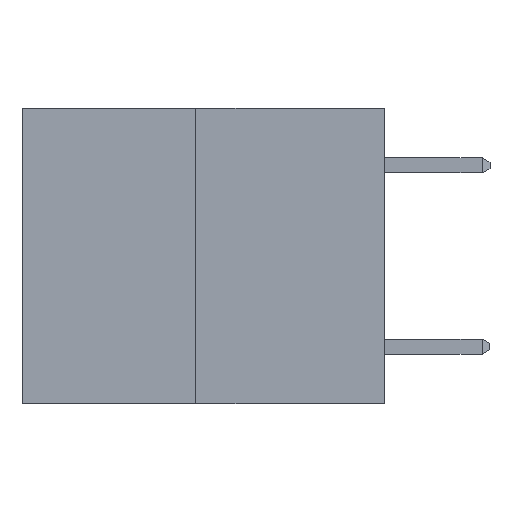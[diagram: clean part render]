
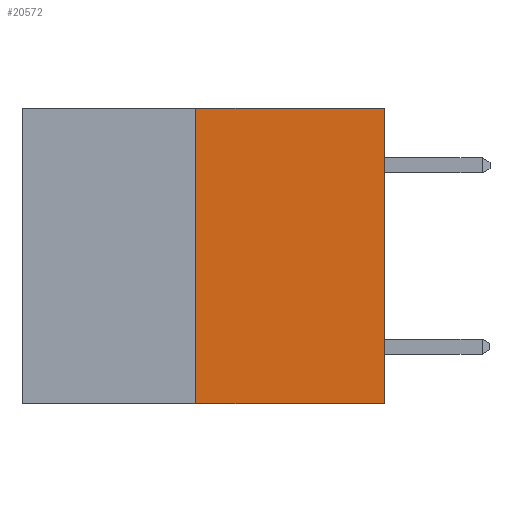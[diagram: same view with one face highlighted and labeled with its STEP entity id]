
A CAD part, left-side view. The second image highlights one B-rep face of the part: STEP entity #20572.
In plain terms, the highlighted planar face has unit normal (-1, 0, 0).
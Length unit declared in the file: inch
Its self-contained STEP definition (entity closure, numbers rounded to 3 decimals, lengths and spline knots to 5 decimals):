
#237 = EDGE_CURVE ( 'NONE', #17981, #3026, #12383, .T. ) ;
#826 = CARTESIAN_POINT ( 'NONE',  ( 0., 0.312, -0.49 ) ) ;
#1086 = AXIS2_PLACEMENT_3D ( 'NONE', #9680, #3223, #11369 ) ;
#1556 = PLANE ( 'NONE',  #1086 ) ;
#3026 = VERTEX_POINT ( 'NONE', #20534 ) ;
#3223 = DIRECTION ( 'NONE',  ( 1., 0., 0. ) ) ;
#3263 = ORIENTED_EDGE ( 'NONE', *, *, #14878, .T. ) ;
#3732 = DIRECTION ( 'NONE',  ( 0., -1., 0. ) ) ;
#4095 = EDGE_CURVE ( 'NONE', #17981, #12749, #14603, .T. ) ;
#4225 = FACE_OUTER_BOUND ( 'NONE', #7385, .T. ) ;
#4967 = VECTOR ( 'NONE', #19743, 39.37008 ) ;
#5757 = LINE ( 'NONE', #15315, #6266 ) ;
#6266 = VECTOR ( 'NONE', #8860, 39.37008 ) ;
#7365 = ORIENTED_EDGE ( 'NONE', *, *, #10284, .F. ) ;
#7385 = EDGE_LOOP ( 'NONE', ( #20879, #19993, #3263, #7365 ) ) ;
#7649 = CARTESIAN_POINT ( 'NONE',  ( 0., 0., 0. ) ) ;
#7756 = VECTOR ( 'NONE', #3732, 39.37008 ) ;
#8355 = CARTESIAN_POINT ( 'NONE',  ( 0., 0.6, -0.49 ) ) ;
#8860 = DIRECTION ( 'NONE',  ( 0., 0., 1. ) ) ;
#8983 = VECTOR ( 'NONE', #16795, 39.37008 ) ;
#9680 = CARTESIAN_POINT ( 'NONE',  ( 0., 0.6, 0. ) ) ;
#10284 = EDGE_CURVE ( 'NONE', #12749, #20030, #11975, .T. ) ;
#11369 = DIRECTION ( 'NONE',  ( 0., 0., -1. ) ) ;
#11975 = LINE ( 'NONE', #20272, #7756 ) ;
#12383 = LINE ( 'NONE', #8355, #8983 ) ;
#12749 = VERTEX_POINT ( 'NONE', #16152 ) ;
#14603 = LINE ( 'NONE', #21181, #4967 ) ;
#14878 = EDGE_CURVE ( 'NONE', #3026, #20030, #5757, .T. ) ;
#15315 = CARTESIAN_POINT ( 'NONE',  ( 0., 0., 0. ) ) ;
#16152 = CARTESIAN_POINT ( 'NONE',  ( 0., 0.312, 0. ) ) ;
#16795 = DIRECTION ( 'NONE',  ( 0., -1., 0. ) ) ;
#17981 = VERTEX_POINT ( 'NONE', #826 ) ;
#19743 = DIRECTION ( 'NONE',  ( 0., 0., 1. ) ) ;
#19993 = ORIENTED_EDGE ( 'NONE', *, *, #237, .T. ) ;
#20030 = VERTEX_POINT ( 'NONE', #7649 ) ;
#20272 = CARTESIAN_POINT ( 'NONE',  ( 0., 0.6, 0. ) ) ;
#20534 = CARTESIAN_POINT ( 'NONE',  ( 0., 0., -0.49 ) ) ;
#20572 = ADVANCED_FACE ( 'NONE', ( #4225 ), #1556, .F. ) ;
#20879 = ORIENTED_EDGE ( 'NONE', *, *, #4095, .F. ) ;
#21181 = CARTESIAN_POINT ( 'NONE',  ( 0., 0.312, -0.49 ) ) ;
